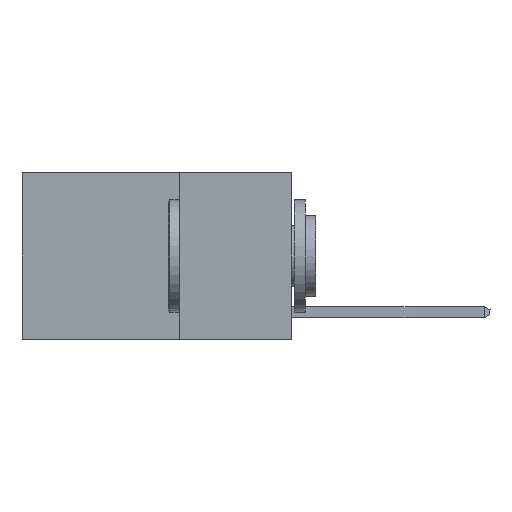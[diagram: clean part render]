
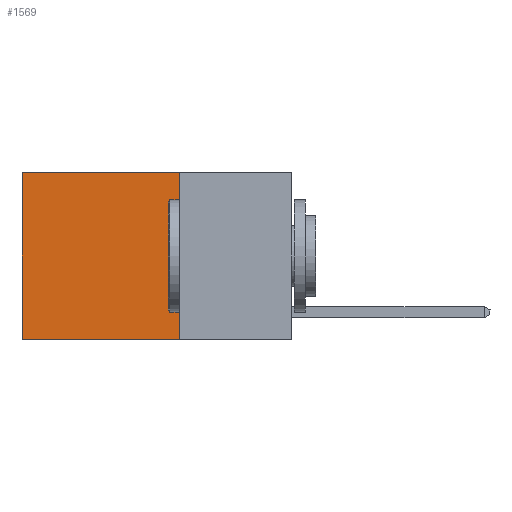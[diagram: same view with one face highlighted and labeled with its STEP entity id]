
A CAD part, left-side view. The second image highlights one B-rep face of the part: STEP entity #1569.
In plain terms, the highlighted planar face has unit normal (-1, 0, 0).
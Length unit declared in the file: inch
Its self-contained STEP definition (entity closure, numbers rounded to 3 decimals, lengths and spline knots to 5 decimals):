
#342 = LINE ( 'NONE', #2588, #3194 ) ;
#903 = EDGE_CURVE ( 'NONE', #11751, #2822, #9916, .T. ) ;
#936 = DIRECTION ( 'NONE',  ( 0., 0., -1. ) ) ;
#1047 = DIRECTION ( 'NONE',  ( 1., 0., 0. ) ) ;
#1165 = CARTESIAN_POINT ( 'NONE',  ( 0.2625, 0.25, 0. ) ) ;
#1288 = CARTESIAN_POINT ( 'NONE',  ( 0.2625, 0.6, 0. ) ) ;
#1505 = DIRECTION ( 'NONE',  ( 0., 0., -1. ) ) ;
#1569 = ADVANCED_FACE ( 'NONE', ( #10066 ), #6476, .F. ) ;
#1861 = LINE ( 'NONE', #5949, #9659 ) ;
#2588 = CARTESIAN_POINT ( 'NONE',  ( 0.2625, 0.25, 0. ) ) ;
#2703 = VERTEX_POINT ( 'NONE', #1288 ) ;
#2822 = VERTEX_POINT ( 'NONE', #9644 ) ;
#3194 = VECTOR ( 'NONE', #10008, 39.37008 ) ;
#3672 = CARTESIAN_POINT ( 'NONE',  ( 0.2625, 0.25, 0. ) ) ;
#5949 = CARTESIAN_POINT ( 'NONE',  ( 0.2625, 0.6, 0. ) ) ;
#6476 = PLANE ( 'NONE',  #11504 ) ;
#6785 = VECTOR ( 'NONE', #9265, 39.37008 ) ;
#6932 = CARTESIAN_POINT ( 'NONE',  ( 0.2625, 0.25, 0. ) ) ;
#7820 = VERTEX_POINT ( 'NONE', #6932 ) ;
#8163 = ORIENTED_EDGE ( 'NONE', *, *, #9495, .T. ) ;
#8169 = ORIENTED_EDGE ( 'NONE', *, *, #903, .F. ) ;
#9220 = CARTESIAN_POINT ( 'NONE',  ( 0.2625, 0.25, -0.37 ) ) ;
#9265 = DIRECTION ( 'NONE',  ( 0., 1., 0. ) ) ;
#9304 = EDGE_LOOP ( 'NONE', ( #8163, #8169, #9438, #9340 ) ) ;
#9340 = ORIENTED_EDGE ( 'NONE', *, *, #10485, .T. ) ;
#9438 = ORIENTED_EDGE ( 'NONE', *, *, #12207, .F. ) ;
#9495 = EDGE_CURVE ( 'NONE', #2703, #2822, #1861, .T. ) ;
#9644 = CARTESIAN_POINT ( 'NONE',  ( 0.2625, 0.6, -0.37 ) ) ;
#9659 = VECTOR ( 'NONE', #10180, 39.37008 ) ;
#9771 = VECTOR ( 'NONE', #1505, 39.37008 ) ;
#9916 = LINE ( 'NONE', #10324, #6785 ) ;
#10008 = DIRECTION ( 'NONE',  ( 0., 1., 0. ) ) ;
#10066 = FACE_OUTER_BOUND ( 'NONE', #9304, .T. ) ;
#10180 = DIRECTION ( 'NONE',  ( 0., 0., -1. ) ) ;
#10324 = CARTESIAN_POINT ( 'NONE',  ( 0.2625, 0.25, -0.37 ) ) ;
#10485 = EDGE_CURVE ( 'NONE', #7820, #2703, #342, .T. ) ;
#11504 = AXIS2_PLACEMENT_3D ( 'NONE', #1165, #1047, #936 ) ;
#11751 = VERTEX_POINT ( 'NONE', #9220 ) ;
#12207 = EDGE_CURVE ( 'NONE', #7820, #11751, #12217, .T. ) ;
#12217 = LINE ( 'NONE', #3672, #9771 ) ;
